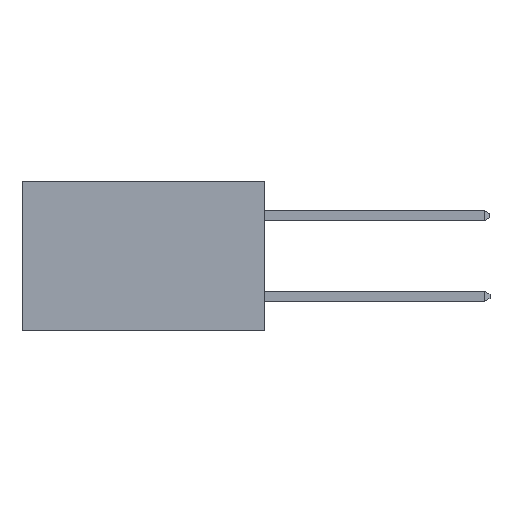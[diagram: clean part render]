
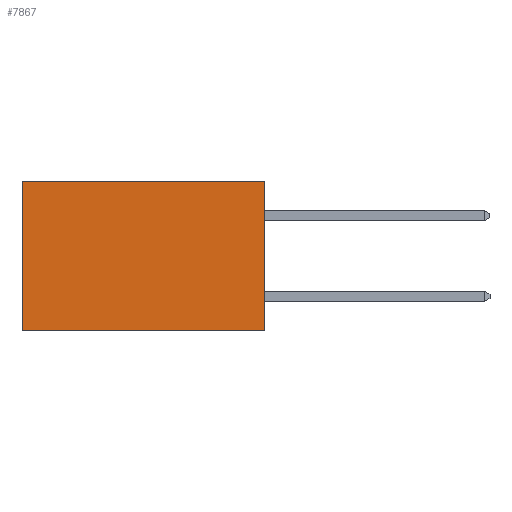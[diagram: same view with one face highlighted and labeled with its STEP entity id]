
A CAD part, left-side view. The second image highlights one B-rep face of the part: STEP entity #7867.
In plain terms, the highlighted planar face has unit normal (-1, 0, 0).
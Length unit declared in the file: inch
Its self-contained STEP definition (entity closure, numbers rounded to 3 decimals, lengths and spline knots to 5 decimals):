
#196 = AXIS2_PLACEMENT_3D ( 'NONE', #5761, #3251, #9096 ) ;
#227 = ORIENTED_EDGE ( 'NONE', *, *, #11217, .F. ) ;
#911 = ORIENTED_EDGE ( 'NONE', *, *, #4424, .T. ) ;
#934 = ORIENTED_EDGE ( 'NONE', *, *, #8436, .F. ) ;
#1342 = LINE ( 'NONE', #8173, #9930 ) ;
#1550 = VERTEX_POINT ( 'NONE', #6143 ) ;
#1769 = CARTESIAN_POINT ( 'NONE',  ( 0.2615, 0.6, -0.37 ) ) ;
#1932 = CARTESIAN_POINT ( 'NONE',  ( 0.2615, 0., -0.37 ) ) ;
#2357 = EDGE_LOOP ( 'NONE', ( #9559, #227, #934, #911 ) ) ;
#2832 = LINE ( 'NONE', #7949, #7020 ) ;
#2853 = DIRECTION ( 'NONE',  ( 0., 1., 0. ) ) ;
#2961 = EDGE_CURVE ( 'NONE', #1550, #9437, #1342, .T. ) ;
#3251 = DIRECTION ( 'NONE',  ( 1., 0., 0. ) ) ;
#3581 = VERTEX_POINT ( 'NONE', #10235 ) ;
#4424 = EDGE_CURVE ( 'NONE', #3581, #1550, #2832, .T. ) ;
#4428 = VERTEX_POINT ( 'NONE', #6279 ) ;
#5516 = FACE_OUTER_BOUND ( 'NONE', #2357, .T. ) ;
#5761 = CARTESIAN_POINT ( 'NONE',  ( 0.2615, 0., -0.37 ) ) ;
#6143 = CARTESIAN_POINT ( 'NONE',  ( 0.2615, 0.6, 0. ) ) ;
#6279 = CARTESIAN_POINT ( 'NONE',  ( 0.2615, 0., -0.37 ) ) ;
#6326 = DIRECTION ( 'NONE',  ( 0., 1., 0. ) ) ;
#6561 = VECTOR ( 'NONE', #2853, 39.37008 ) ;
#7020 = VECTOR ( 'NONE', #6326, 39.37008 ) ;
#7867 = ADVANCED_FACE ( 'NONE', ( #5516 ), #8257, .F. ) ;
#7949 = CARTESIAN_POINT ( 'NONE',  ( 0.2615, 0., 0. ) ) ;
#8121 = VECTOR ( 'NONE', #8858, 39.37008 ) ;
#8123 = DIRECTION ( 'NONE',  ( 0., 0., -1. ) ) ;
#8173 = CARTESIAN_POINT ( 'NONE',  ( 0.2615, 0.6, -0.37 ) ) ;
#8257 = PLANE ( 'NONE',  #196 ) ;
#8436 = EDGE_CURVE ( 'NONE', #3581, #4428, #10381, .T. ) ;
#8858 = DIRECTION ( 'NONE',  ( 0., 0., -1. ) ) ;
#9096 = DIRECTION ( 'NONE',  ( 0., 0., -1. ) ) ;
#9437 = VERTEX_POINT ( 'NONE', #1769 ) ;
#9559 = ORIENTED_EDGE ( 'NONE', *, *, #2961, .T. ) ;
#9713 = CARTESIAN_POINT ( 'NONE',  ( 0.2615, 0., -0.37 ) ) ;
#9930 = VECTOR ( 'NONE', #8123, 39.37008 ) ;
#10235 = CARTESIAN_POINT ( 'NONE',  ( 0.2615, 0., 0. ) ) ;
#10381 = LINE ( 'NONE', #9713, #8121 ) ;
#10992 = LINE ( 'NONE', #1932, #6561 ) ;
#11217 = EDGE_CURVE ( 'NONE', #4428, #9437, #10992, .T. ) ;
